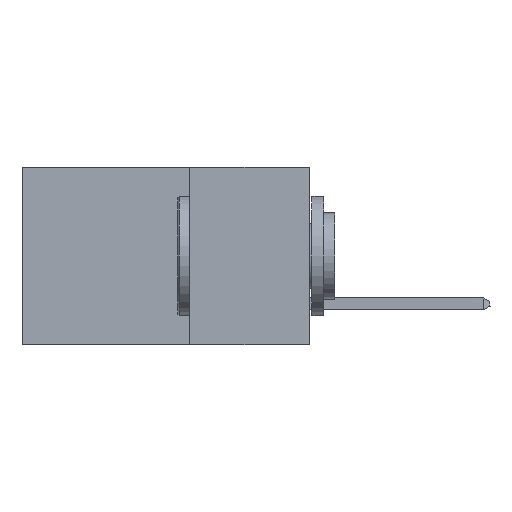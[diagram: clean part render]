
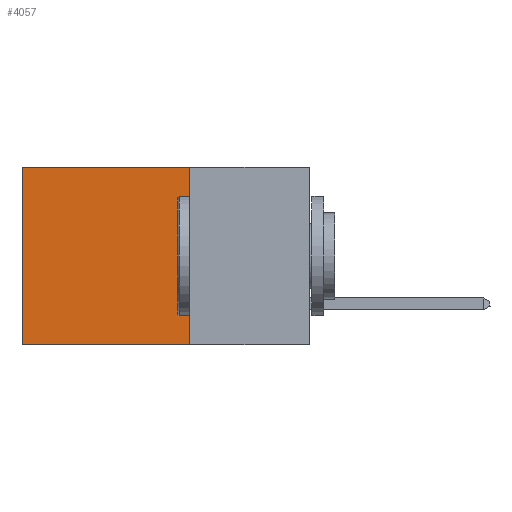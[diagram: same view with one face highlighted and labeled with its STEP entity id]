
A CAD part, left-side view. The second image highlights one B-rep face of the part: STEP entity #4057.
In plain terms, the highlighted planar face has unit normal (-1, 0, 0).
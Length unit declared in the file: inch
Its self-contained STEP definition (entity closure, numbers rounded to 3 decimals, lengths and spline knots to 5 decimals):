
#820 = ORIENTED_EDGE ( 'NONE', *, *, #19887, .F. ) ;
#1117 = VECTOR ( 'NONE', #18316, 39.37008 ) ;
#1118 = DIRECTION ( 'NONE',  ( 0., 1., 0. ) ) ;
#2675 = AXIS2_PLACEMENT_3D ( 'NONE', #10349, #10522, #16166 ) ;
#3544 = FACE_OUTER_BOUND ( 'NONE', #19049, .T. ) ;
#4057 = ADVANCED_FACE ( 'NONE', ( #3544 ), #15902, .F. ) ;
#4656 = CARTESIAN_POINT ( 'NONE',  ( 0.2875, 0.6, -0.37 ) ) ;
#5166 = EDGE_CURVE ( 'NONE', #7815, #24145, #6244, .T. ) ;
#6244 = LINE ( 'NONE', #24663, #21736 ) ;
#6270 = LINE ( 'NONE', #19957, #1117 ) ;
#7285 = ORIENTED_EDGE ( 'NONE', *, *, #10518, .T. ) ;
#7815 = VERTEX_POINT ( 'NONE', #9642 ) ;
#9409 = CARTESIAN_POINT ( 'NONE',  ( 0.2875, 0.6, 0. ) ) ;
#9642 = CARTESIAN_POINT ( 'NONE',  ( 0.2875, 0.25, -0.37 ) ) ;
#10220 = DIRECTION ( 'NONE',  ( 0., 0., -1. ) ) ;
#10349 = CARTESIAN_POINT ( 'NONE',  ( 0.2875, 0.25, 0. ) ) ;
#10518 = EDGE_CURVE ( 'NONE', #14495, #24145, #19726, .T. ) ;
#10522 = DIRECTION ( 'NONE',  ( 1., 0., 0. ) ) ;
#13638 = EDGE_CURVE ( 'NONE', #18095, #14495, #6270, .T. ) ;
#14063 = VECTOR ( 'NONE', #10220, 39.37008 ) ;
#14370 = LINE ( 'NONE', #20086, #14063 ) ;
#14495 = VERTEX_POINT ( 'NONE', #20607 ) ;
#15780 = ORIENTED_EDGE ( 'NONE', *, *, #5166, .F. ) ;
#15902 = PLANE ( 'NONE',  #2675 ) ;
#16166 = DIRECTION ( 'NONE',  ( 0., 0., -1. ) ) ;
#18095 = VERTEX_POINT ( 'NONE', #23074 ) ;
#18316 = DIRECTION ( 'NONE',  ( 0., 1., 0. ) ) ;
#19049 = EDGE_LOOP ( 'NONE', ( #7285, #15780, #820, #19813 ) ) ;
#19726 = LINE ( 'NONE', #9409, #20035 ) ;
#19813 = ORIENTED_EDGE ( 'NONE', *, *, #13638, .T. ) ;
#19887 = EDGE_CURVE ( 'NONE', #18095, #7815, #14370, .T. ) ;
#19957 = CARTESIAN_POINT ( 'NONE',  ( 0.2875, 0.25, 0. ) ) ;
#20035 = VECTOR ( 'NONE', #23078, 39.37008 ) ;
#20086 = CARTESIAN_POINT ( 'NONE',  ( 0.2875, 0.25, 0. ) ) ;
#20607 = CARTESIAN_POINT ( 'NONE',  ( 0.2875, 0.6, 0. ) ) ;
#21736 = VECTOR ( 'NONE', #1118, 39.37008 ) ;
#23074 = CARTESIAN_POINT ( 'NONE',  ( 0.2875, 0.25, 0. ) ) ;
#23078 = DIRECTION ( 'NONE',  ( 0., 0., -1. ) ) ;
#24145 = VERTEX_POINT ( 'NONE', #4656 ) ;
#24663 = CARTESIAN_POINT ( 'NONE',  ( 0.2875, 0.25, -0.37 ) ) ;
